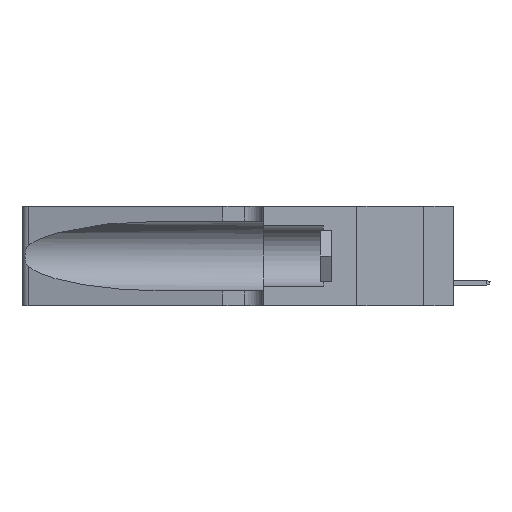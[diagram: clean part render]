
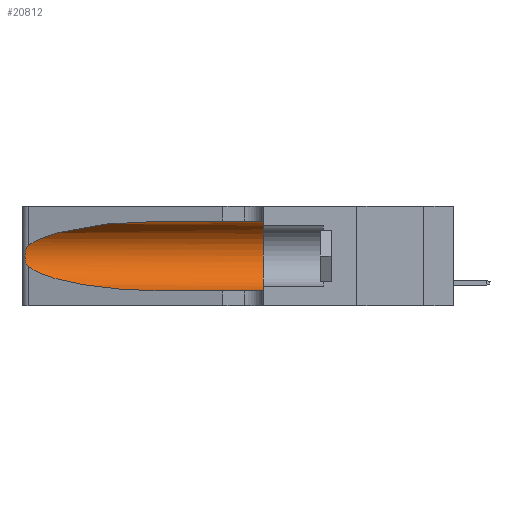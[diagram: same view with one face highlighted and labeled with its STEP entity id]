
A CAD part, left-side view. The second image highlights one B-rep face of the part: STEP entity #20812.
In plain terms, the highlighted cylindrical face has radius 3.308 mm (diameter 6.617 mm), a partial arc.
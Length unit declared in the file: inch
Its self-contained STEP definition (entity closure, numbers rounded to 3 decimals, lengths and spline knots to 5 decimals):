
#415 = CARTESIAN_POINT ( 'NONE',  ( 0.1305, 1.61858, 0.05475 ) ) ;
#725 = CARTESIAN_POINT ( 'NONE',  ( 0.25487, 1.22718, 0.22369 ) ) ;
#901 = CARTESIAN_POINT ( 'NONE',  ( 0.1305, 0.35, 0.05475 ) ) ;
#1344 = DIRECTION ( 'NONE',  ( 0., 1., 0. ) ) ;
#2737 = EDGE_CURVE ( 'NONE', #32114, #12635, #27223, .T. ) ;
#3590 = AXIS2_PLACEMENT_3D ( 'NONE', #14952, #1344, #6949 ) ;
#4578 = ORIENTED_EDGE ( 'NONE', *, *, #12235, .T. ) ;
#5653 = CARTESIAN_POINT ( 'NONE',  ( 0.1305, 1.61858, 0.31525 ) ) ;
#6022 = VERTEX_POINT ( 'NONE', #901 ) ;
#6147 = B_SPLINE_CURVE_WITH_KNOTS ( 'NONE', 3,
 ( #20548, #7508, #31293, #28993, #34597, #10262, #12696, #34255, #20730, #31483, #10434, #16020, #34433, #29169 ),
 .UNSPECIFIED., .F., .F.,
 ( 4, 2, 2, 2, 2, 2, 4 ),
 ( 0., 0.00027, 0.00053, 0.00107, 0.0016, 0.00187, 0.00214 ),
 .UNSPECIFIED. ) ;
#6384 = CARTESIAN_POINT ( 'NONE',  ( 0.25487, 1.22718, 0.22369 ) ) ;
#6609 = EDGE_CURVE ( 'NONE', #25396, #7319, #21158, .T. ) ;
#6904 = DIRECTION ( 'NONE',  ( 0., -1., 0. ) ) ;
#6949 = DIRECTION ( 'NONE',  ( 0., 0., 1. ) ) ;
#7319 = VERTEX_POINT ( 'NONE', #19725 ) ;
#7508 = CARTESIAN_POINT ( 'NONE',  ( 0.25555, 1.22994, 0.2215 ) ) ;
#7770 = CARTESIAN_POINT ( 'NONE',  ( 0.18966, 0.96281, 0.05475 ) ) ;
#7986 = VECTOR ( 'NONE', #16297, 39.37008 ) ;
#8084 = CARTESIAN_POINT ( 'NONE',  ( 0.1305, 0.72297, 0.31525 ) ) ;
#8572 = CIRCLE ( 'NONE', #3590, 0.13025 ) ;
#8656 = CARTESIAN_POINT ( 'NONE',  ( 0.2373, 1.15595, 0.28018 ) ) ;
#10194 = FACE_OUTER_BOUND ( 'NONE', #26520, .T. ) ;
#10262 = CARTESIAN_POINT ( 'NONE',  ( 0.26018, 1.23835, 0.19895 ) ) ;
#10296 = EDGE_CURVE ( 'NONE', #12635, #25396, #6147, .T. ) ;
#10434 = CARTESIAN_POINT ( 'NONE',  ( 0.25789, 1.23486, 0.15765 ) ) ;
#11916 = EDGE_CURVE ( 'NONE', #29193, #6022, #8572, .T. ) ;
#12235 = EDGE_CURVE ( 'NONE', #7319, #6022, #19439, .T. ) ;
#12489 = CARTESIAN_POINT ( 'NONE',  ( 0.25487, 1.22718, 0.14631 ) ) ;
#12635 = VERTEX_POINT ( 'NONE', #725 ) ;
#12696 = CARTESIAN_POINT ( 'NONE',  ( 0.26075, 1.23896, 0.19203 ) ) ;
#13673 = ORIENTED_EDGE ( 'NONE', *, *, #26152, .F. ) ;
#13861 = DIRECTION ( 'NONE',  ( 0., -1., 0. ) ) ;
#14564 = ORIENTED_EDGE ( 'NONE', *, *, #10296, .T. ) ;
#14952 = CARTESIAN_POINT ( 'NONE',  ( 0.1305, 0.35, 0.185 ) ) ;
#16020 = CARTESIAN_POINT ( 'NONE',  ( 0.25639, 1.23186, 0.15144 ) ) ;
#16297 = DIRECTION ( 'NONE',  ( 0., -1., 0. ) ) ;
#16686 = ORIENTED_EDGE ( 'NONE', *, *, #11916, .F. ) ;
#17876 = CARTESIAN_POINT ( 'NONE',  ( 0.2373, 1.15595, 0.08982 ) ) ;
#19439 = LINE ( 'NONE', #415, #31504 ) ;
#19725 = CARTESIAN_POINT ( 'NONE',  ( 0.1305, 0.72297, 0.05475 ) ) ;
#20548 = CARTESIAN_POINT ( 'NONE',  ( 0.25487, 1.22718, 0.22369 ) ) ;
#20730 = CARTESIAN_POINT ( 'NONE',  ( 0.26017, 1.23833, 0.17102 ) ) ;
#20812 = ADVANCED_FACE ( 'NONE', ( #10194 ), #31217, .F. ) ;
#21158 =( BOUNDED_CURVE ( )  B_SPLINE_CURVE ( 3, ( #31580, #17876, #7770, #28557 ),
 .UNSPECIFIED., .F., .T. ) 
 B_SPLINE_CURVE_WITH_KNOTS ( ( 4, 4 ),
 ( 3.44316, 4.71239 ),
 .UNSPECIFIED. ) 
 CURVE ( )  GEOMETRIC_REPRESENTATION_ITEM ( )  RATIONAL_B_SPLINE_CURVE ( ( 1., 0.87, 0.87, 1. ) ) 
 REPRESENTATION_ITEM ( '' )  );
#22375 = ORIENTED_EDGE ( 'NONE', *, *, #6609, .T. ) ;
#24297 = LINE ( 'NONE', #5653, #7986 ) ;
#24493 = CARTESIAN_POINT ( 'NONE',  ( 0.1305, 0.72297, 0.31525 ) ) ;
#25136 = AXIS2_PLACEMENT_3D ( 'NONE', #34005, #6904, #25549 ) ;
#25396 = VERTEX_POINT ( 'NONE', #12489 ) ;
#25549 = DIRECTION ( 'NONE',  ( 0., 0., -1. ) ) ;
#26152 = EDGE_CURVE ( 'NONE', #32114, #29193, #24297, .T. ) ;
#26520 = EDGE_LOOP ( 'NONE', ( #29098, #14564, #22375, #4578, #16686, #13673 ) ) ;
#27223 =( BOUNDED_CURVE ( )  B_SPLINE_CURVE ( 3, ( #24493, #32630, #8656, #6384 ),
 .UNSPECIFIED., .F., .T. ) 
 B_SPLINE_CURVE_WITH_KNOTS ( ( 4, 4 ),
 ( 1.5708, 2.84003 ),
 .UNSPECIFIED. ) 
 CURVE ( )  GEOMETRIC_REPRESENTATION_ITEM ( )  RATIONAL_B_SPLINE_CURVE ( ( 1., 0.87, 0.87, 1. ) ) 
 REPRESENTATION_ITEM ( '' )  );
#28557 = CARTESIAN_POINT ( 'NONE',  ( 0.1305, 0.72297, 0.05475 ) ) ;
#28993 = CARTESIAN_POINT ( 'NONE',  ( 0.25787, 1.23484, 0.2124 ) ) ;
#29098 = ORIENTED_EDGE ( 'NONE', *, *, #2737, .T. ) ;
#29169 = CARTESIAN_POINT ( 'NONE',  ( 0.25487, 1.22718, 0.14631 ) ) ;
#29193 = VERTEX_POINT ( 'NONE', #29353 ) ;
#29353 = CARTESIAN_POINT ( 'NONE',  ( 0.1305, 0.35, 0.31525 ) ) ;
#31217 = CYLINDRICAL_SURFACE ( 'NONE', #25136, 0.13025 ) ;
#31293 = CARTESIAN_POINT ( 'NONE',  ( 0.25639, 1.23184, 0.21858 ) ) ;
#31483 = CARTESIAN_POINT ( 'NONE',  ( 0.25856, 1.23593, 0.16098 ) ) ;
#31504 = VECTOR ( 'NONE', #13861, 39.37008 ) ;
#31580 = CARTESIAN_POINT ( 'NONE',  ( 0.25487, 1.22718, 0.14631 ) ) ;
#32114 = VERTEX_POINT ( 'NONE', #8084 ) ;
#32630 = CARTESIAN_POINT ( 'NONE',  ( 0.18966, 0.96281, 0.31525 ) ) ;
#34005 = CARTESIAN_POINT ( 'NONE',  ( 0.1305, 1.61858, 0.185 ) ) ;
#34255 = CARTESIAN_POINT ( 'NONE',  ( 0.26075, 1.23896, 0.178 ) ) ;
#34433 = CARTESIAN_POINT ( 'NONE',  ( 0.25555, 1.22993, 0.14849 ) ) ;
#34597 = CARTESIAN_POINT ( 'NONE',  ( 0.25854, 1.2359, 0.20912 ) ) ;
